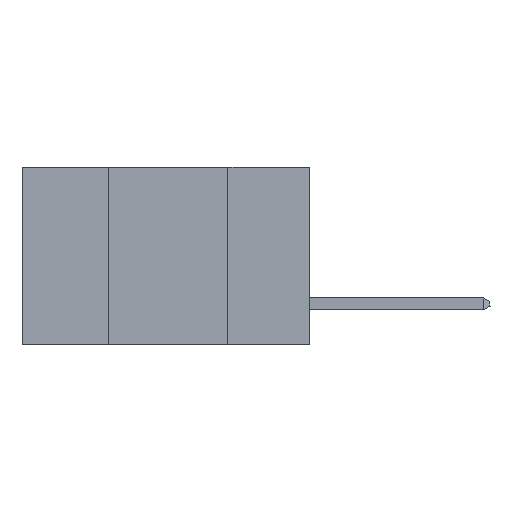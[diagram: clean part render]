
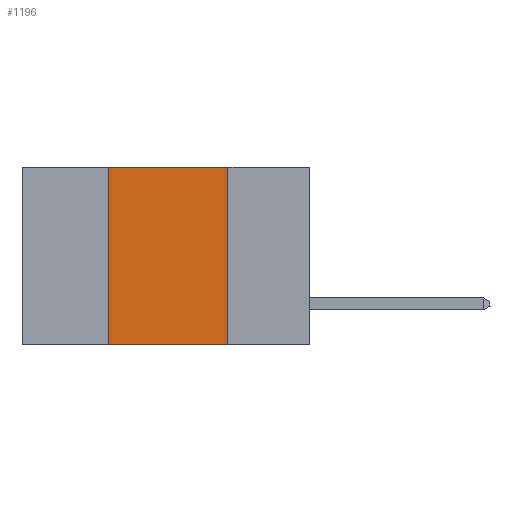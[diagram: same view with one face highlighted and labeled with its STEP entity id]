
A CAD part, left-side view. The second image highlights one B-rep face of the part: STEP entity #1196.
In plain terms, the highlighted planar face has unit normal (-1, 0, 0).
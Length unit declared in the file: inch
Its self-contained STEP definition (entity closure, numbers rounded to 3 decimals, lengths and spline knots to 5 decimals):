
#88 = LINE ( 'NONE', #18353, #15553 ) ;
#126 = PLANE ( 'NONE',  #4123 ) ;
#1160 = CARTESIAN_POINT ( 'NONE',  ( 0., 0.17, -0.37 ) ) ;
#1196 = ADVANCED_FACE ( 'NONE', ( #7937 ), #126, .F. ) ;
#2171 = DIRECTION ( 'NONE',  ( 1., 0., 0. ) ) ;
#3105 = ORIENTED_EDGE ( 'NONE', *, *, #25038, .F. ) ;
#4015 = LINE ( 'NONE', #17596, #16388 ) ;
#4123 = AXIS2_PLACEMENT_3D ( 'NONE', #14023, #2171, #14207 ) ;
#4255 = VERTEX_POINT ( 'NONE', #4908 ) ;
#4908 = CARTESIAN_POINT ( 'NONE',  ( 0., 0.42, -0.37 ) ) ;
#4919 = LINE ( 'NONE', #18774, #9533 ) ;
#5653 = EDGE_LOOP ( 'NONE', ( #9116, #22420, #3105, #24294 ) ) ;
#7731 = VECTOR ( 'NONE', #24187, 39.37008 ) ;
#7937 = FACE_OUTER_BOUND ( 'NONE', #5653, .T. ) ;
#9116 = ORIENTED_EDGE ( 'NONE', *, *, #15894, .F. ) ;
#9156 = VERTEX_POINT ( 'NONE', #19482 ) ;
#9533 = VECTOR ( 'NONE', #15053, 39.37008 ) ;
#9830 = EDGE_CURVE ( 'NONE', #12394, #9156, #4015, .T. ) ;
#12394 = VERTEX_POINT ( 'NONE', #16267 ) ;
#14023 = CARTESIAN_POINT ( 'NONE',  ( 0., 0.6, 0. ) ) ;
#14207 = DIRECTION ( 'NONE',  ( 0., 0., -1. ) ) ;
#15053 = DIRECTION ( 'NONE',  ( 0., -1., 0. ) ) ;
#15553 = VECTOR ( 'NONE', #18608, 39.37008 ) ;
#15697 = DIRECTION ( 'NONE',  ( 0., -1., 0. ) ) ;
#15894 = EDGE_CURVE ( 'NONE', #9156, #22441, #88, .T. ) ;
#16267 = CARTESIAN_POINT ( 'NONE',  ( 0., 0.42, 0. ) ) ;
#16388 = VECTOR ( 'NONE', #15697, 39.37008 ) ;
#17596 = CARTESIAN_POINT ( 'NONE',  ( 0., 0.6, 0. ) ) ;
#18353 = CARTESIAN_POINT ( 'NONE',  ( 0., 0.17, 0. ) ) ;
#18608 = DIRECTION ( 'NONE',  ( 0., 0., -1. ) ) ;
#18774 = CARTESIAN_POINT ( 'NONE',  ( 0., 0.6, -0.37 ) ) ;
#19482 = CARTESIAN_POINT ( 'NONE',  ( 0., 0.17, 0. ) ) ;
#21025 = LINE ( 'NONE', #23927, #7731 ) ;
#22420 = ORIENTED_EDGE ( 'NONE', *, *, #9830, .F. ) ;
#22441 = VERTEX_POINT ( 'NONE', #1160 ) ;
#23927 = CARTESIAN_POINT ( 'NONE',  ( 0., 0.42, 0. ) ) ;
#24187 = DIRECTION ( 'NONE',  ( 0., 0., 1. ) ) ;
#24294 = ORIENTED_EDGE ( 'NONE', *, *, #24825, .T. ) ;
#24825 = EDGE_CURVE ( 'NONE', #4255, #22441, #4919, .T. ) ;
#25038 = EDGE_CURVE ( 'NONE', #4255, #12394, #21025, .T. ) ;
